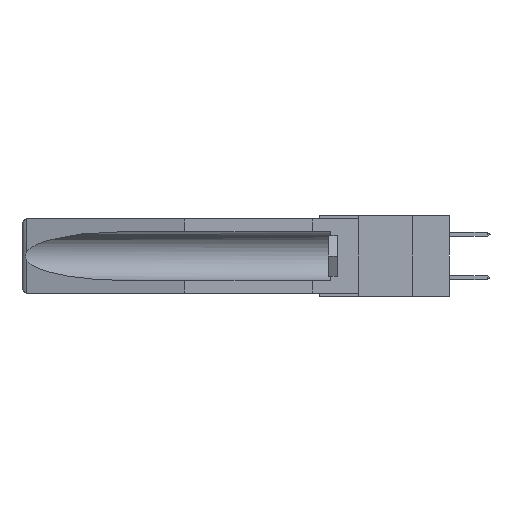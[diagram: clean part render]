
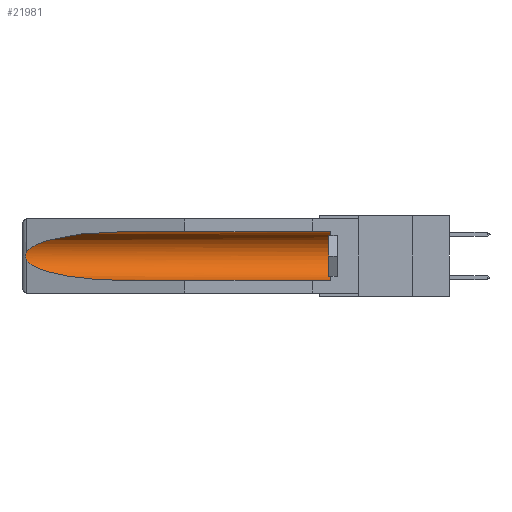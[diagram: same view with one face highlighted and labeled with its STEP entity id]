
A CAD part, left-side view. The second image highlights one B-rep face of the part: STEP entity #21981.
In plain terms, the highlighted cylindrical face has radius 2.857 mm (diameter 5.715 mm), a partial arc.
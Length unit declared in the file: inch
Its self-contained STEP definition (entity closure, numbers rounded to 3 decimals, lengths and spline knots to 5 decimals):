
#776 = CARTESIAN_POINT ( 'NONE',  ( 0.155, 1.07973, -0.059 ) ) ;
#1360 = EDGE_CURVE ( 'NONE', #13816, #25900, #13000, .T. ) ;
#1368 = VERTEX_POINT ( 'NONE', #1914 ) ;
#1465 = CARTESIAN_POINT ( 'NONE',  ( 0.155, -0.30754, -0.284 ) ) ;
#1814 = DIRECTION ( 'NONE',  ( 0., -1., 0. ) ) ;
#1914 = CARTESIAN_POINT ( 'NONE',  ( 0.26537, 1.52718, -0.14972 ) ) ;
#2044 = CARTESIAN_POINT ( 'NONE',  ( 0.2673, 1.53269, -0.17917 ) ) ;
#2117 = AXIS2_PLACEMENT_3D ( 'NONE', #17807, #1814, #17717 ) ;
#4081 =( BOUNDED_CURVE ( )  B_SPLINE_CURVE ( 3, ( #776, #6846, #6494, #22803 ),
 .UNSPECIFIED., .F., .F. ) 
 B_SPLINE_CURVE_WITH_KNOTS ( ( 4, 4 ),
 ( 4.71239, 6.08839 ),
 .UNSPECIFIED. ) 
 CURVE ( )  GEOMETRIC_REPRESENTATION_ITEM ( )  RATIONAL_B_SPLINE_CURVE ( ( 1., 0.848, 0.848, 1. ) ) 
 REPRESENTATION_ITEM ( '' )  );
#5425 = CARTESIAN_POINT ( 'NONE',  ( 0.26537, 1.52718, -0.19328 ) ) ;
#5671 = EDGE_CURVE ( 'NONE', #25900, #23191, #14298, .T. ) ;
#5890 = EDGE_CURVE ( 'NONE', #1368, #21199, #17532, .T. ) ;
#6337 = ORIENTED_EDGE ( 'NONE', *, *, #16200, .F. ) ;
#6494 = CARTESIAN_POINT ( 'NONE',  ( 0.25451, 1.48313, -0.09465 ) ) ;
#6846 = CARTESIAN_POINT ( 'NONE',  ( 0.21114, 1.30732, -0.059 ) ) ;
#7364 = ORIENTED_EDGE ( 'NONE', *, *, #1360, .T. ) ;
#8245 = AXIS2_PLACEMENT_3D ( 'NONE', #17856, #11708, #9499 ) ;
#8316 = CARTESIAN_POINT ( 'NONE',  ( 0.26537, 1.52718, -0.19328 ) ) ;
#8638 = CARTESIAN_POINT ( 'NONE',  ( 0.155, 1.07973, -0.284 ) ) ;
#9124 =( BOUNDED_CURVE ( )  B_SPLINE_CURVE ( 3, ( #20524, #24515, #25433, #15415 ),
 .UNSPECIFIED., .F., .F. ) 
 B_SPLINE_CURVE_WITH_KNOTS ( ( 4, 4 ),
 ( 0.1948, 1.5708 ),
 .UNSPECIFIED. ) 
 CURVE ( )  GEOMETRIC_REPRESENTATION_ITEM ( )  RATIONAL_B_SPLINE_CURVE ( ( 1., 0.848, 0.848, 1. ) ) 
 REPRESENTATION_ITEM ( '' )  );
#9499 = DIRECTION ( 'NONE',  ( 0., 0., 1. ) ) ;
#10033 = CARTESIAN_POINT ( 'NONE',  ( 0.2673, 1.5327, -0.16383 ) ) ;
#10122 = CARTESIAN_POINT ( 'NONE',  ( 0.26597, 1.5296, -0.19026 ) ) ;
#10402 = VECTOR ( 'NONE', #19689, 39.37008 ) ;
#10925 = DIRECTION ( 'NONE',  ( 0., 1., 0. ) ) ;
#11708 = DIRECTION ( 'NONE',  ( 0., 1., 0. ) ) ;
#12329 = CARTESIAN_POINT ( 'NONE',  ( 0.26655, 1.53094, -0.18657 ) ) ;
#13000 = CIRCLE ( 'NONE', #2117, 0.1125 ) ;
#13359 = CARTESIAN_POINT ( 'NONE',  ( 0.155, 1.07973, -0.059 ) ) ;
#13816 = VERTEX_POINT ( 'NONE', #26169 ) ;
#14083 = CARTESIAN_POINT ( 'NONE',  ( 0.2675, 1.53308, -0.16763 ) ) ;
#14298 = LINE ( 'NONE', #23260, #20962 ) ;
#15370 = ORIENTED_EDGE ( 'NONE', *, *, #5890, .T. ) ;
#15415 = CARTESIAN_POINT ( 'NONE',  ( 0.155, 1.07973, -0.284 ) ) ;
#15628 = ORIENTED_EDGE ( 'NONE', *, *, #5671, .T. ) ;
#16200 = EDGE_CURVE ( 'NONE', #13816, #20493, #25893, .T. ) ;
#17532 = B_SPLINE_CURVE_WITH_KNOTS ( 'NONE', 3,
 ( #26038, #22107, #19358, #10033, #14083, #20167, #2044, #12329, #10122, #8316 ),
 .UNSPECIFIED., .F., .F.,
 ( 4, 2, 2, 2, 4 ),
 ( 0., 0.00029, 0.00058, 0.00087, 0.00117 ),
 .UNSPECIFIED. ) ;
#17717 = DIRECTION ( 'NONE',  ( 0., 0., 1. ) ) ;
#17807 = CARTESIAN_POINT ( 'NONE',  ( 0.155, 0.126, -0.1715 ) ) ;
#17856 = CARTESIAN_POINT ( 'NONE',  ( 0.155, -0.30754, -0.1715 ) ) ;
#19358 = CARTESIAN_POINT ( 'NONE',  ( 0.26654, 1.53092, -0.15636 ) ) ;
#19381 = CYLINDRICAL_SURFACE ( 'NONE', #8245, 0.1125 ) ;
#19689 = DIRECTION ( 'NONE',  ( 0., 1., 0. ) ) ;
#20028 = FACE_OUTER_BOUND ( 'NONE', #24165, .T. ) ;
#20167 = CARTESIAN_POINT ( 'NONE',  ( 0.2675, 1.53308, -0.17534 ) ) ;
#20493 = VERTEX_POINT ( 'NONE', #8638 ) ;
#20524 = CARTESIAN_POINT ( 'NONE',  ( 0.26537, 1.52718, -0.19328 ) ) ;
#20962 = VECTOR ( 'NONE', #10925, 39.37008 ) ;
#21199 = VERTEX_POINT ( 'NONE', #5425 ) ;
#21560 = EDGE_CURVE ( 'NONE', #23191, #1368, #4081, .T. ) ;
#21981 = ADVANCED_FACE ( 'NONE', ( #20028 ), #19381, .F. ) ;
#22107 = CARTESIAN_POINT ( 'NONE',  ( 0.26597, 1.52961, -0.15275 ) ) ;
#22737 = CARTESIAN_POINT ( 'NONE',  ( 0.155, 0.126, -0.059 ) ) ;
#22803 = CARTESIAN_POINT ( 'NONE',  ( 0.26537, 1.52718, -0.14972 ) ) ;
#22935 = ORIENTED_EDGE ( 'NONE', *, *, #24411, .T. ) ;
#23191 = VERTEX_POINT ( 'NONE', #13359 ) ;
#23260 = CARTESIAN_POINT ( 'NONE',  ( 0.155, -0.30754, -0.059 ) ) ;
#24165 = EDGE_LOOP ( 'NONE', ( #25854, #15370, #22935, #6337, #7364, #15628 ) ) ;
#24411 = EDGE_CURVE ( 'NONE', #21199, #20493, #9124, .T. ) ;
#24515 = CARTESIAN_POINT ( 'NONE',  ( 0.25451, 1.48313, -0.24835 ) ) ;
#25433 = CARTESIAN_POINT ( 'NONE',  ( 0.21114, 1.30732, -0.284 ) ) ;
#25854 = ORIENTED_EDGE ( 'NONE', *, *, #21560, .T. ) ;
#25893 = LINE ( 'NONE', #1465, #10402 ) ;
#25900 = VERTEX_POINT ( 'NONE', #22737 ) ;
#26038 = CARTESIAN_POINT ( 'NONE',  ( 0.26537, 1.52718, -0.14972 ) ) ;
#26169 = CARTESIAN_POINT ( 'NONE',  ( 0.155, 0.126, -0.284 ) ) ;
